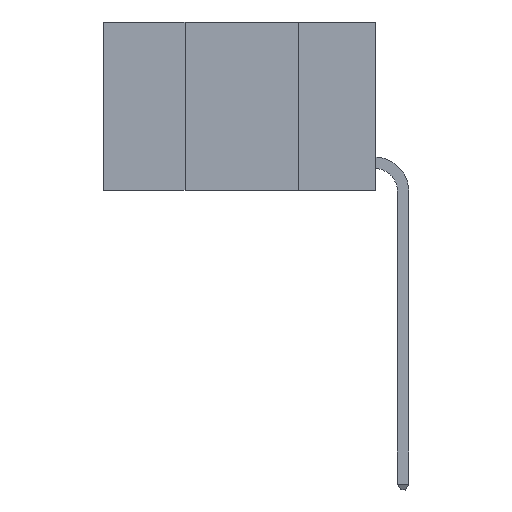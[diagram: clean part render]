
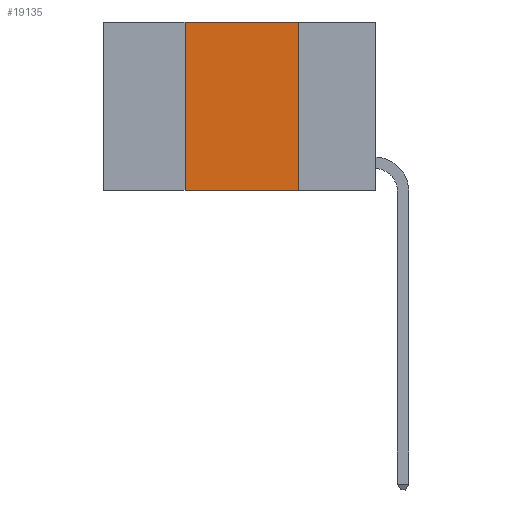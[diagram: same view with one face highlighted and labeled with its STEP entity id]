
A CAD part, left-side view. The second image highlights one B-rep face of the part: STEP entity #19135.
In plain terms, the highlighted planar face has unit normal (-1, 0, 0).
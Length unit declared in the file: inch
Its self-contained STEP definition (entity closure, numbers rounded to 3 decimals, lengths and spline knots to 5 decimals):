
#256 = VECTOR ( 'NONE', #16086, 39.37008 ) ;
#984 = DIRECTION ( 'NONE',  ( 0., -1., 0. ) ) ;
#1120 = AXIS2_PLACEMENT_3D ( 'NONE', #8433, #16038, #6996 ) ;
#1319 = ORIENTED_EDGE ( 'NONE', *, *, #14855, .F. ) ;
#2574 = VECTOR ( 'NONE', #13365, 39.37008 ) ;
#2764 = CARTESIAN_POINT ( 'NONE',  ( 0., 0.17, 0. ) ) ;
#3736 = EDGE_LOOP ( 'NONE', ( #15277, #1319, #16475, #12491 ) ) ;
#5448 = PLANE ( 'NONE',  #1120 ) ;
#5918 = CARTESIAN_POINT ( 'NONE',  ( 0., 0.17, -0.37 ) ) ;
#6394 = CARTESIAN_POINT ( 'NONE',  ( 0., 0.42, 0. ) ) ;
#6907 = CARTESIAN_POINT ( 'NONE',  ( 0., 0.42, -0.37 ) ) ;
#6996 = DIRECTION ( 'NONE',  ( 0., 0., -1. ) ) ;
#7866 = VECTOR ( 'NONE', #984, 39.37008 ) ;
#8208 = CARTESIAN_POINT ( 'NONE',  ( 0., 0.42, 0. ) ) ;
#8433 = CARTESIAN_POINT ( 'NONE',  ( 0., 0.6, 0. ) ) ;
#8557 = CARTESIAN_POINT ( 'NONE',  ( 0., 0.6, 0. ) ) ;
#9130 = FACE_OUTER_BOUND ( 'NONE', #3736, .T. ) ;
#9835 = VERTEX_POINT ( 'NONE', #5918 ) ;
#10370 = LINE ( 'NONE', #8208, #16474 ) ;
#10690 = LINE ( 'NONE', #16372, #2574 ) ;
#11330 = EDGE_CURVE ( 'NONE', #16523, #9835, #11925, .T. ) ;
#11668 = CARTESIAN_POINT ( 'NONE',  ( 0., 0.6, -0.37 ) ) ;
#11688 = VERTEX_POINT ( 'NONE', #6394 ) ;
#11925 = LINE ( 'NONE', #11668, #7866 ) ;
#12491 = ORIENTED_EDGE ( 'NONE', *, *, #11330, .T. ) ;
#12937 = LINE ( 'NONE', #8557, #256 ) ;
#13343 = EDGE_CURVE ( 'NONE', #16523, #11688, #10370, .T. ) ;
#13365 = DIRECTION ( 'NONE',  ( 0., 0., -1. ) ) ;
#14321 = VERTEX_POINT ( 'NONE', #2764 ) ;
#14855 = EDGE_CURVE ( 'NONE', #11688, #14321, #12937, .T. ) ;
#15277 = ORIENTED_EDGE ( 'NONE', *, *, #17350, .F. ) ;
#16038 = DIRECTION ( 'NONE',  ( 1., 0., 0. ) ) ;
#16086 = DIRECTION ( 'NONE',  ( 0., -1., 0. ) ) ;
#16372 = CARTESIAN_POINT ( 'NONE',  ( 0., 0.17, 0. ) ) ;
#16474 = VECTOR ( 'NONE', #17175, 39.37008 ) ;
#16475 = ORIENTED_EDGE ( 'NONE', *, *, #13343, .F. ) ;
#16523 = VERTEX_POINT ( 'NONE', #6907 ) ;
#17175 = DIRECTION ( 'NONE',  ( 0., 0., 1. ) ) ;
#17350 = EDGE_CURVE ( 'NONE', #14321, #9835, #10690, .T. ) ;
#19135 = ADVANCED_FACE ( 'NONE', ( #9130 ), #5448, .F. ) ;
